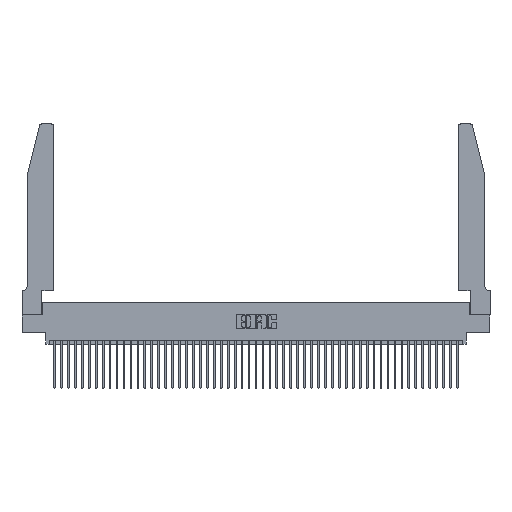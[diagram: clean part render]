
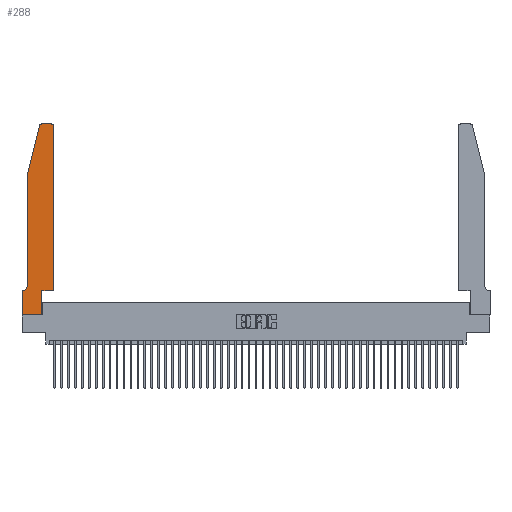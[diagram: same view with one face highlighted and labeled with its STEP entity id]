
A CAD part, top view. The second image highlights one B-rep face of the part: STEP entity #288.
In plain terms, the highlighted planar face has unit normal (0, 0, 1).
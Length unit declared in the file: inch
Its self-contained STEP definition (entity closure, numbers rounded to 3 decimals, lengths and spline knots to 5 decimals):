
#288 = ADVANCED_FACE ( 'NONE', ( #9842 ), #5827, .T. ) ;
#451 = ORIENTED_EDGE ( 'NONE', *, *, #30453, .T. ) ;
#715 = EDGE_CURVE ( 'NONE', #35302, #41966, #44019, .T. ) ;
#1287 = CIRCLE ( 'NONE', #10671, 0.03 ) ;
#1989 = EDGE_CURVE ( 'NONE', #12838, #20666, #20134, .T. ) ;
#2380 = VERTEX_POINT ( 'NONE', #17368 ) ;
#2458 = DIRECTION ( 'NONE',  ( 0., 1., 0. ) ) ;
#2491 = VECTOR ( 'NONE', #40229, 39.37008 ) ;
#3068 = DIRECTION ( 'NONE',  ( 1., 0., 0. ) ) ;
#3316 = CARTESIAN_POINT ( 'NONE',  ( 0.0755, 0.35, 0.37 ) ) ;
#3401 = ORIENTED_EDGE ( 'NONE', *, *, #1989, .T. ) ;
#3577 = LINE ( 'NONE', #7256, #41387 ) ;
#3769 = VECTOR ( 'NONE', #6508, 39.37008 ) ;
#3854 = VECTOR ( 'NONE', #37804, 39.37008 ) ;
#3894 = CARTESIAN_POINT ( 'NONE',  ( 0.4505, 0.35, 0.37 ) ) ;
#5064 = DIRECTION ( 'NONE',  ( 0., 0., 1. ) ) ;
#5253 = VECTOR ( 'NONE', #46571, 39.37008 ) ;
#5355 = CARTESIAN_POINT ( 'NONE',  ( 0., 0., 0.37 ) ) ;
#5827 = PLANE ( 'NONE',  #35047 ) ;
#6508 = DIRECTION ( 'NONE',  ( -1., 0., 0. ) ) ;
#6630 = EDGE_CURVE ( 'NONE', #21660, #37254, #14389, .T. ) ;
#6733 = EDGE_CURVE ( 'NONE', #19556, #11879, #7245, .T. ) ;
#6818 = CARTESIAN_POINT ( 'NONE',  ( 0.4205, 2.75, 0.37 ) ) ;
#7245 = CIRCLE ( 'NONE', #37783, 0.03 ) ;
#7256 = CARTESIAN_POINT ( 'NONE',  ( 0.0755, 2., 0.37 ) ) ;
#8361 = EDGE_CURVE ( 'NONE', #47944, #46570, #23478, .T. ) ;
#8393 = ORIENTED_EDGE ( 'NONE', *, *, #715, .T. ) ;
#8428 = ORIENTED_EDGE ( 'NONE', *, *, #30228, .T. ) ;
#8940 = CARTESIAN_POINT ( 'NONE',  ( 0.4205, 2.72, 0.37 ) ) ;
#9683 = CARTESIAN_POINT ( 'NONE',  ( 0.25487, 2.72718, 0.37 ) ) ;
#9842 = FACE_OUTER_BOUND ( 'NONE', #10699, .T. ) ;
#10048 = EDGE_CURVE ( 'NONE', #41966, #2380, #48704, .T. ) ;
#10217 = CARTESIAN_POINT ( 'NONE',  ( 0.0755, 2., 0.37 ) ) ;
#10671 = AXIS2_PLACEMENT_3D ( 'NONE', #25800, #33856, #3068 ) ;
#10699 = EDGE_LOOP ( 'NONE', ( #29492, #26340, #29975, #17745, #8393, #47689, #31933, #3401, #8428, #28956, #451, #38726 ) ) ;
#10953 = CARTESIAN_POINT ( 'NONE',  ( 0.4505, 0.35, 0.37 ) ) ;
#11879 = VERTEX_POINT ( 'NONE', #6818 ) ;
#12838 = VERTEX_POINT ( 'NONE', #22667 ) ;
#13179 = DIRECTION ( 'NONE',  ( 0., 0., 1. ) ) ;
#14109 = EDGE_CURVE ( 'NONE', #37254, #35302, #3577, .T. ) ;
#14389 = LINE ( 'NONE', #10217, #2491 ) ;
#15210 = CARTESIAN_POINT ( 'NONE',  ( 0.2865, 0., 0.37 ) ) ;
#15957 = EDGE_CURVE ( 'NONE', #2380, #12838, #29648, .T. ) ;
#17098 = CARTESIAN_POINT ( 'NONE',  ( 0.2865, 0.35, 0.37 ) ) ;
#17328 = VECTOR ( 'NONE', #25517, 39.37008 ) ;
#17368 = CARTESIAN_POINT ( 'NONE',  ( 0., 0.35, 0.37 ) ) ;
#17745 = ORIENTED_EDGE ( 'NONE', *, *, #14109, .T. ) ;
#19275 = AXIS2_PLACEMENT_3D ( 'NONE', #27945, #43175, #20630 ) ;
#19556 = VERTEX_POINT ( 'NONE', #47702 ) ;
#19662 = VECTOR ( 'NONE', #26222, 39.37008 ) ;
#19700 = CARTESIAN_POINT ( 'NONE',  ( 0.0055, 0.35, 0.37 ) ) ;
#19728 = CARTESIAN_POINT ( 'NONE',  ( 0., 0., 0.37 ) ) ;
#19996 = DIRECTION ( 'NONE',  ( 1., 0., 0. ) ) ;
#20134 = LINE ( 'NONE', #19728, #5253 ) ;
#20630 = DIRECTION ( 'NONE',  ( -1., 0., 0. ) ) ;
#20666 = VERTEX_POINT ( 'NONE', #15210 ) ;
#20902 = CARTESIAN_POINT ( 'NONE',  ( 0.2865, 0.35, 0.37 ) ) ;
#21660 = VERTEX_POINT ( 'NONE', #9683 ) ;
#22008 = LINE ( 'NONE', #45120, #19662 ) ;
#22176 = CARTESIAN_POINT ( 'NONE',  ( 0.284, 2.75, 0.37 ) ) ;
#22667 = CARTESIAN_POINT ( 'NONE',  ( 0., 0., 0.37 ) ) ;
#23268 = LINE ( 'NONE', #10953, #17328 ) ;
#23478 = LINE ( 'NONE', #3894, #3854 ) ;
#25517 = DIRECTION ( 'NONE',  ( 0., 1., 0. ) ) ;
#25800 = CARTESIAN_POINT ( 'NONE',  ( 0.284, 2.72, 0.37 ) ) ;
#26222 = DIRECTION ( 'NONE',  ( -1., 0., 0. ) ) ;
#26340 = ORIENTED_EDGE ( 'NONE', *, *, #40070, .T. ) ;
#27945 = CARTESIAN_POINT ( 'NONE',  ( 0.0055, 0.42, 0.37 ) ) ;
#28722 = CARTESIAN_POINT ( 'NONE',  ( 0., 0.35, 0.37 ) ) ;
#28891 = DIRECTION ( 'NONE',  ( 1., 0., 0. ) ) ;
#28909 = CARTESIAN_POINT ( 'NONE',  ( 0.4505, 0.35, 0.37 ) ) ;
#28956 = ORIENTED_EDGE ( 'NONE', *, *, #8361, .T. ) ;
#29492 = ORIENTED_EDGE ( 'NONE', *, *, #34163, .T. ) ;
#29648 = LINE ( 'NONE', #5355, #43149 ) ;
#29975 = ORIENTED_EDGE ( 'NONE', *, *, #6630, .T. ) ;
#30228 = EDGE_CURVE ( 'NONE', #20666, #47944, #36274, .T. ) ;
#30453 = EDGE_CURVE ( 'NONE', #46570, #19556, #23268, .T. ) ;
#31933 = ORIENTED_EDGE ( 'NONE', *, *, #15957, .T. ) ;
#33856 = DIRECTION ( 'NONE',  ( 0., 0., 1. ) ) ;
#34163 = EDGE_CURVE ( 'NONE', #11879, #47352, #22008, .T. ) ;
#34171 = DIRECTION ( 'NONE',  ( 0., -1., 0. ) ) ;
#35047 = AXIS2_PLACEMENT_3D ( 'NONE', #28722, #13179, #28891 ) ;
#35098 = VECTOR ( 'NONE', #2458, 39.37008 ) ;
#35302 = VERTEX_POINT ( 'NONE', #47330 ) ;
#35639 = DIRECTION ( 'NONE',  ( 0., -1., 0. ) ) ;
#36274 = LINE ( 'NONE', #17098, #35098 ) ;
#37254 = VERTEX_POINT ( 'NONE', #44398 ) ;
#37783 = AXIS2_PLACEMENT_3D ( 'NONE', #8940, #5064, #19996 ) ;
#37804 = DIRECTION ( 'NONE',  ( 1., 0., 0. ) ) ;
#38726 = ORIENTED_EDGE ( 'NONE', *, *, #6733, .T. ) ;
#40070 = EDGE_CURVE ( 'NONE', #47352, #21660, #1287, .T. ) ;
#40229 = DIRECTION ( 'NONE',  ( -0.239, -0.971, 0. ) ) ;
#41387 = VECTOR ( 'NONE', #34171, 39.37008 ) ;
#41966 = VERTEX_POINT ( 'NONE', #19700 ) ;
#43149 = VECTOR ( 'NONE', #35639, 39.37008 ) ;
#43175 = DIRECTION ( 'NONE',  ( 0., 0., -1. ) ) ;
#44019 = CIRCLE ( 'NONE', #19275, 0.07 ) ;
#44398 = CARTESIAN_POINT ( 'NONE',  ( 0.0755, 2., 0.37 ) ) ;
#45120 = CARTESIAN_POINT ( 'NONE',  ( 0.2605, 2.75, 0.37 ) ) ;
#46570 = VERTEX_POINT ( 'NONE', #28909 ) ;
#46571 = DIRECTION ( 'NONE',  ( 1., 0., 0. ) ) ;
#47330 = CARTESIAN_POINT ( 'NONE',  ( 0.0755, 0.42, 0.37 ) ) ;
#47352 = VERTEX_POINT ( 'NONE', #22176 ) ;
#47689 = ORIENTED_EDGE ( 'NONE', *, *, #10048, .T. ) ;
#47702 = CARTESIAN_POINT ( 'NONE',  ( 0.4505, 2.72, 0.37 ) ) ;
#47944 = VERTEX_POINT ( 'NONE', #20902 ) ;
#48704 = LINE ( 'NONE', #3316, #3769 ) ;
